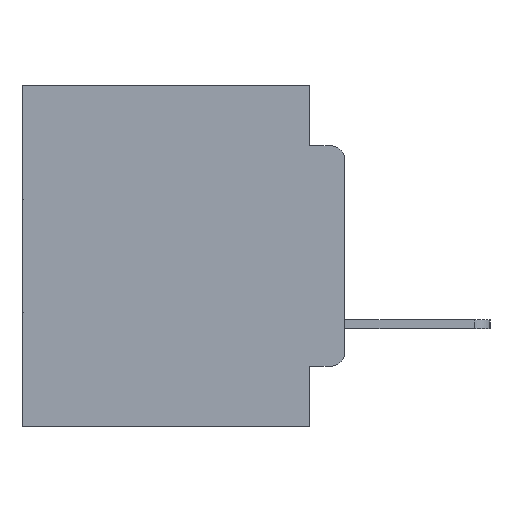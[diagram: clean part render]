
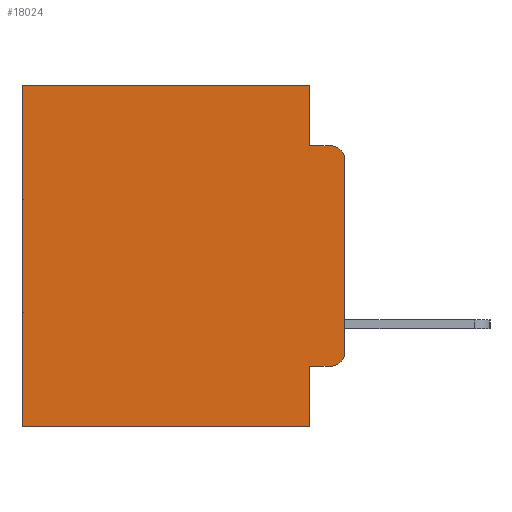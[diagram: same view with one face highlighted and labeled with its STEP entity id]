
A CAD part, left-side view. The second image highlights one B-rep face of the part: STEP entity #18024.
In plain terms, the highlighted planar face has unit normal (-1, 0, 0).
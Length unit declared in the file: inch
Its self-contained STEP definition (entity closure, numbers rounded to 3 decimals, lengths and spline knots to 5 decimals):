
#668 = EDGE_LOOP ( 'NONE', ( #29422, #5973, #12226, #19183, #25066, #2761, #27755, #4192, #23382, #29092 ) ) ;
#938 = EDGE_CURVE ( 'NONE', #8459, #21367, #27653, .T. ) ;
#1089 = DIRECTION ( 'NONE',  ( 0., -1., 0. ) ) ;
#1146 = VERTEX_POINT ( 'NONE', #27667 ) ;
#1238 = VERTEX_POINT ( 'NONE', #20079 ) ;
#1460 = DIRECTION ( 'NONE',  ( 0., 0., -1. ) ) ;
#1538 = VECTOR ( 'NONE', #8923, 39.37008 ) ;
#2341 = VECTOR ( 'NONE', #1089, 39.37008 ) ;
#2761 = ORIENTED_EDGE ( 'NONE', *, *, #21729, .T. ) ;
#3239 = DIRECTION ( 'NONE',  ( 0., 0., -1. ) ) ;
#4183 = VERTEX_POINT ( 'NONE', #11701 ) ;
#4192 = ORIENTED_EDGE ( 'NONE', *, *, #20229, .F. ) ;
#4278 = CARTESIAN_POINT ( 'NONE',  ( 0.298, 0.473, 0. ) ) ;
#4529 = VERTEX_POINT ( 'NONE', #19073 ) ;
#4795 = DIRECTION ( 'NONE',  ( 0., 0., -1. ) ) ;
#4825 = LINE ( 'NONE', #12451, #16514 ) ;
#4827 = LINE ( 'NONE', #22371, #23986 ) ;
#5433 = DIRECTION ( 'NONE',  ( 0., 0., -1. ) ) ;
#5796 = EDGE_CURVE ( 'NONE', #11527, #12019, #22300, .T. ) ;
#5973 = ORIENTED_EDGE ( 'NONE', *, *, #938, .T. ) ;
#6504 = CARTESIAN_POINT ( 'NONE',  ( 0.298, 0., -0.5 ) ) ;
#7176 = EDGE_CURVE ( 'NONE', #8459, #15755, #4827, .T. ) ;
#7684 = CARTESIAN_POINT ( 'NONE',  ( 0.298, 0., -0.3915 ) ) ;
#7733 = LINE ( 'NONE', #6504, #1538 ) ;
#8459 = VERTEX_POINT ( 'NONE', #16726 ) ;
#8496 = LINE ( 'NONE', #21895, #2341 ) ;
#8885 = AXIS2_PLACEMENT_3D ( 'NONE', #18605, #28851, #4795 ) ;
#8923 = DIRECTION ( 'NONE',  ( 0., 1., 0. ) ) ;
#10649 = DIRECTION ( 'NONE',  ( 1., 0., 0. ) ) ;
#10670 = CARTESIAN_POINT ( 'NONE',  ( 0.298, 0.02, -0.3915 ) ) ;
#10858 = EDGE_CURVE ( 'NONE', #4183, #15755, #13626, .T. ) ;
#11154 = LINE ( 'NONE', #19439, #23420 ) ;
#11527 = VERTEX_POINT ( 'NONE', #23365 ) ;
#11701 = CARTESIAN_POINT ( 'NONE',  ( 0.298, 0.02, -0.4115 ) ) ;
#12019 = VERTEX_POINT ( 'NONE', #4278 ) ;
#12226 = ORIENTED_EDGE ( 'NONE', *, *, #27560, .F. ) ;
#12436 = EDGE_CURVE ( 'NONE', #15497, #4183, #8496, .T. ) ;
#12451 = CARTESIAN_POINT ( 'NONE',  ( 0.298, 0.051, -0.0885 ) ) ;
#12723 = VECTOR ( 'NONE', #3239, 39.37008 ) ;
#13012 = DIRECTION ( 'NONE',  ( 0., 0., -1. ) ) ;
#13626 = CIRCLE ( 'NONE', #25420, 0.02 ) ;
#14339 = CARTESIAN_POINT ( 'NONE',  ( 0.298, 0.051, 0. ) ) ;
#14929 = CARTESIAN_POINT ( 'NONE',  ( 0.298, 0.051, 0. ) ) ;
#15497 = VERTEX_POINT ( 'NONE', #24912 ) ;
#15755 = VERTEX_POINT ( 'NONE', #7684 ) ;
#15802 = FACE_OUTER_BOUND ( 'NONE', #668, .T. ) ;
#16514 = VECTOR ( 'NONE', #21745, 39.37008 ) ;
#16726 = CARTESIAN_POINT ( 'NONE',  ( 0.298, 0., -0.1085 ) ) ;
#17435 = LINE ( 'NONE', #14339, #22793 ) ;
#18024 = ADVANCED_FACE ( 'NONE', ( #15802 ), #26499, .F. ) ;
#18605 = CARTESIAN_POINT ( 'NONE',  ( 0.298, 0.02, -0.1085 ) ) ;
#19073 = CARTESIAN_POINT ( 'NONE',  ( 0.298, 0.051, -0.5 ) ) ;
#19183 = ORIENTED_EDGE ( 'NONE', *, *, #23238, .F. ) ;
#19439 = CARTESIAN_POINT ( 'NONE',  ( 0.298, 0.473, 0. ) ) ;
#19697 = LINE ( 'NONE', #14929, #12723 ) ;
#20079 = CARTESIAN_POINT ( 'NONE',  ( 0.298, 0.473, -0.5 ) ) ;
#20117 = CARTESIAN_POINT ( 'NONE',  ( 0.298, 0.02, -0.0885 ) ) ;
#20229 = EDGE_CURVE ( 'NONE', #15497, #4529, #19697, .T. ) ;
#21195 = DIRECTION ( 'NONE',  ( 0., 0., -1. ) ) ;
#21367 = VERTEX_POINT ( 'NONE', #20117 ) ;
#21729 = EDGE_CURVE ( 'NONE', #12019, #1238, #11154, .T. ) ;
#21745 = DIRECTION ( 'NONE',  ( 0., -1., 0. ) ) ;
#21895 = CARTESIAN_POINT ( 'NONE',  ( 0.298, 0.051, -0.4115 ) ) ;
#22300 = LINE ( 'NONE', #23127, #27365 ) ;
#22371 = CARTESIAN_POINT ( 'NONE',  ( 0.298, 0., 0. ) ) ;
#22793 = VECTOR ( 'NONE', #21195, 39.37008 ) ;
#23127 = CARTESIAN_POINT ( 'NONE',  ( 0.298, 0., 0. ) ) ;
#23238 = EDGE_CURVE ( 'NONE', #11527, #1146, #17435, .T. ) ;
#23365 = CARTESIAN_POINT ( 'NONE',  ( 0.298, 0.051, 0. ) ) ;
#23382 = ORIENTED_EDGE ( 'NONE', *, *, #12436, .T. ) ;
#23420 = VECTOR ( 'NONE', #5433, 39.37008 ) ;
#23986 = VECTOR ( 'NONE', #1460, 39.37008 ) ;
#24427 = CARTESIAN_POINT ( 'NONE',  ( 0.298, 0., 0. ) ) ;
#24912 = CARTESIAN_POINT ( 'NONE',  ( 0.298, 0.051, -0.4115 ) ) ;
#25066 = ORIENTED_EDGE ( 'NONE', *, *, #5796, .T. ) ;
#25420 = AXIS2_PLACEMENT_3D ( 'NONE', #10670, #26602, #13012 ) ;
#26431 = AXIS2_PLACEMENT_3D ( 'NONE', #24427, #10649, #26580 ) ;
#26499 = PLANE ( 'NONE',  #26431 ) ;
#26580 = DIRECTION ( 'NONE',  ( 0., 0., -1. ) ) ;
#26602 = DIRECTION ( 'NONE',  ( -1., 0., 0. ) ) ;
#27365 = VECTOR ( 'NONE', #29060, 39.37008 ) ;
#27560 = EDGE_CURVE ( 'NONE', #1146, #21367, #4825, .T. ) ;
#27653 = CIRCLE ( 'NONE', #8885, 0.02 ) ;
#27667 = CARTESIAN_POINT ( 'NONE',  ( 0.298, 0.051, -0.0885 ) ) ;
#27755 = ORIENTED_EDGE ( 'NONE', *, *, #27939, .F. ) ;
#27939 = EDGE_CURVE ( 'NONE', #4529, #1238, #7733, .T. ) ;
#28851 = DIRECTION ( 'NONE',  ( -1., 0., 0. ) ) ;
#29060 = DIRECTION ( 'NONE',  ( 0., 1., 0. ) ) ;
#29092 = ORIENTED_EDGE ( 'NONE', *, *, #10858, .T. ) ;
#29422 = ORIENTED_EDGE ( 'NONE', *, *, #7176, .F. ) ;
